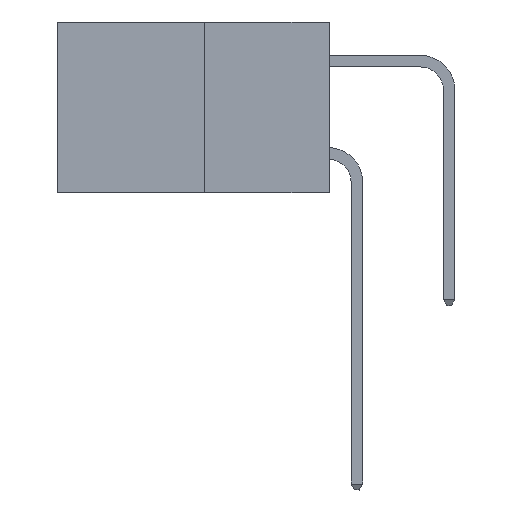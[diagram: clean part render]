
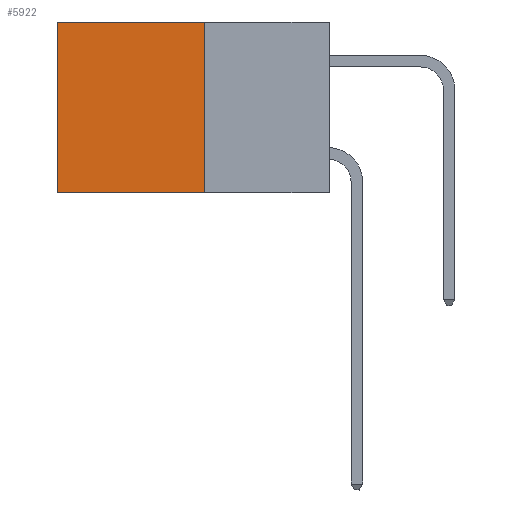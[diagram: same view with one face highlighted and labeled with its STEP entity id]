
A CAD part, left-side view. The second image highlights one B-rep face of the part: STEP entity #5922.
In plain terms, the highlighted planar face has unit normal (-1, 0, 0).
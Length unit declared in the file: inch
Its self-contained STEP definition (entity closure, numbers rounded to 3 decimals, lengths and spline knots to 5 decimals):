
#108 = VECTOR ( 'NONE', #12495, 39.37008 ) ;
#1027 = VERTEX_POINT ( 'NONE', #8880 ) ;
#1353 = VERTEX_POINT ( 'NONE', #16878 ) ;
#1408 = CARTESIAN_POINT ( 'NONE',  ( 0.277, 0.59, -0.37 ) ) ;
#3723 = DIRECTION ( 'NONE',  ( 0., 1., 0. ) ) ;
#4444 = EDGE_CURVE ( 'NONE', #10292, #18809, #12010, .T. ) ;
#5922 = ADVANCED_FACE ( 'NONE', ( #15827 ), #9716, .F. ) ;
#7285 = VECTOR ( 'NONE', #12681, 39.37008 ) ;
#7783 = VECTOR ( 'NONE', #3723, 39.37008 ) ;
#7892 = CARTESIAN_POINT ( 'NONE',  ( 0.277, 0.27, 0. ) ) ;
#8428 = LINE ( 'NONE', #1408, #16341 ) ;
#8880 = CARTESIAN_POINT ( 'NONE',  ( 0.277, 0.59, -0.37 ) ) ;
#9002 = CARTESIAN_POINT ( 'NONE',  ( 0.277, 0.27, 0. ) ) ;
#9643 = DIRECTION ( 'NONE',  ( 0., 0., -1. ) ) ;
#9716 = PLANE ( 'NONE',  #13430 ) ;
#10159 = CARTESIAN_POINT ( 'NONE',  ( 0.277, 0.27, -0.37 ) ) ;
#10292 = VERTEX_POINT ( 'NONE', #9002 ) ;
#10998 = EDGE_CURVE ( 'NONE', #1353, #1027, #8428, .T. ) ;
#12010 = LINE ( 'NONE', #12426, #108 ) ;
#12426 = CARTESIAN_POINT ( 'NONE',  ( 0.277, 0.27, -0.37 ) ) ;
#12495 = DIRECTION ( 'NONE',  ( 0., 0., -1. ) ) ;
#12626 = ORIENTED_EDGE ( 'NONE', *, *, #14361, .T. ) ;
#12681 = DIRECTION ( 'NONE',  ( 0., 1., 0. ) ) ;
#13430 = AXIS2_PLACEMENT_3D ( 'NONE', #10159, #18013, #9643 ) ;
#13623 = EDGE_LOOP ( 'NONE', ( #18065, #15547, #14536, #12626 ) ) ;
#14361 = EDGE_CURVE ( 'NONE', #10292, #1353, #15730, .T. ) ;
#14536 = ORIENTED_EDGE ( 'NONE', *, *, #4444, .F. ) ;
#14979 = CARTESIAN_POINT ( 'NONE',  ( 0.277, 0.27, -0.37 ) ) ;
#15547 = ORIENTED_EDGE ( 'NONE', *, *, #18946, .F. ) ;
#15730 = LINE ( 'NONE', #7892, #7285 ) ;
#15827 = FACE_OUTER_BOUND ( 'NONE', #13623, .T. ) ;
#16341 = VECTOR ( 'NONE', #18899, 39.37008 ) ;
#16878 = CARTESIAN_POINT ( 'NONE',  ( 0.277, 0.59, 0. ) ) ;
#18013 = DIRECTION ( 'NONE',  ( 1., 0., 0. ) ) ;
#18065 = ORIENTED_EDGE ( 'NONE', *, *, #10998, .T. ) ;
#18809 = VERTEX_POINT ( 'NONE', #19148 ) ;
#18899 = DIRECTION ( 'NONE',  ( 0., 0., -1. ) ) ;
#18946 = EDGE_CURVE ( 'NONE', #18809, #1027, #19767, .T. ) ;
#19148 = CARTESIAN_POINT ( 'NONE',  ( 0.277, 0.27, -0.37 ) ) ;
#19767 = LINE ( 'NONE', #14979, #7783 ) ;
